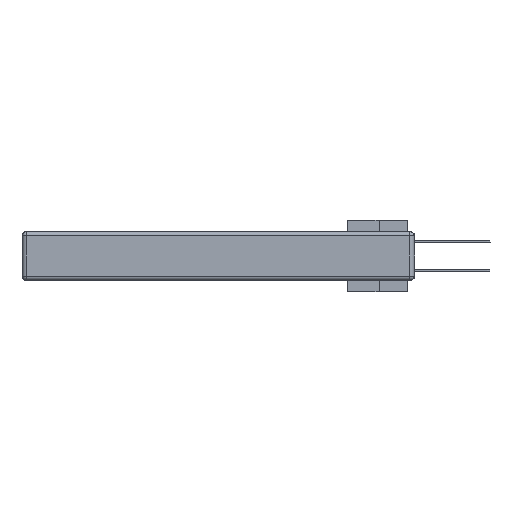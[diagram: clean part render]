
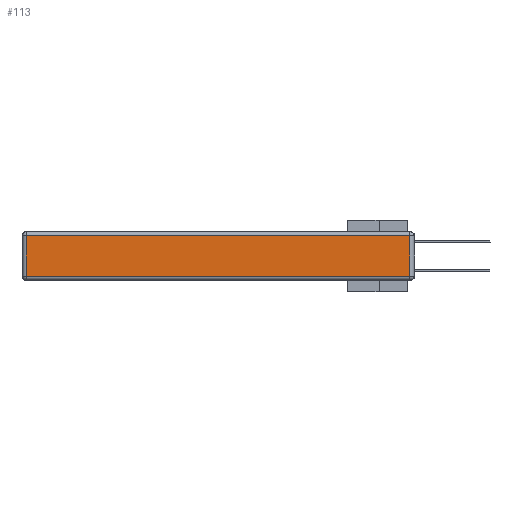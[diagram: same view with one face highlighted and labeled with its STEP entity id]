
A CAD part, left-side view. The second image highlights one B-rep face of the part: STEP entity #113.
In plain terms, the highlighted planar face has unit normal (-1, 0, 0).
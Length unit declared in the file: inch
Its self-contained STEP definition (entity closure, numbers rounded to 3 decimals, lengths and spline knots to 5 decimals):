
#113 = ADVANCED_FACE ( 'NONE', ( #27626 ), #10174, .T. ) ;
#1454 = VERTEX_POINT ( 'NONE', #16090 ) ;
#2201 = AXIS2_PLACEMENT_3D ( 'NONE', #15465, #24579, #2639 ) ;
#2639 = DIRECTION ( 'NONE',  ( 0., 0., 1. ) ) ;
#3125 = DIRECTION ( 'NONE',  ( 0., 0., -1. ) ) ;
#3153 = DIRECTION ( 'NONE',  ( 0., 0., 1. ) ) ;
#3309 = LINE ( 'NONE', #20299, #27949 ) ;
#3883 = CARTESIAN_POINT ( 'NONE',  ( 0., 0.03, -0.03 ) ) ;
#4058 = VERTEX_POINT ( 'NONE', #22180 ) ;
#5304 = ORIENTED_EDGE ( 'NONE', *, *, #15159, .T. ) ;
#5862 = CARTESIAN_POINT ( 'NONE',  ( 0., 2.72, -0.343 ) ) ;
#7704 = CARTESIAN_POINT ( 'NONE',  ( 0., 2.72, -0.313 ) ) ;
#10174 = PLANE ( 'NONE',  #2201 ) ;
#10340 = LINE ( 'NONE', #17716, #16652 ) ;
#10435 = VERTEX_POINT ( 'NONE', #3883 ) ;
#11179 = CARTESIAN_POINT ( 'NONE',  ( 0., 2.75, -0.03 ) ) ;
#12518 = ORIENTED_EDGE ( 'NONE', *, *, #18437, .T. ) ;
#12753 = VECTOR ( 'NONE', #3125, 39.37008 ) ;
#14022 = EDGE_LOOP ( 'NONE', ( #29431, #5304, #17447, #12518 ) ) ;
#14356 = EDGE_CURVE ( 'NONE', #19228, #4058, #10340, .T. ) ;
#15159 = EDGE_CURVE ( 'NONE', #4058, #10435, #3309, .T. ) ;
#15465 = CARTESIAN_POINT ( 'NONE',  ( 0., 0., -0.343 ) ) ;
#16090 = CARTESIAN_POINT ( 'NONE',  ( 0., 2.72, -0.03 ) ) ;
#16652 = VECTOR ( 'NONE', #27465, 39.37008 ) ;
#17447 = ORIENTED_EDGE ( 'NONE', *, *, #31294, .T. ) ;
#17716 = CARTESIAN_POINT ( 'NONE',  ( 0., 0., -0.313 ) ) ;
#18437 = EDGE_CURVE ( 'NONE', #1454, #19228, #22518, .T. ) ;
#19228 = VERTEX_POINT ( 'NONE', #7704 ) ;
#20299 = CARTESIAN_POINT ( 'NONE',  ( 0., 0.03, -0.343 ) ) ;
#22180 = CARTESIAN_POINT ( 'NONE',  ( 0., 0.03, -0.313 ) ) ;
#22518 = LINE ( 'NONE', #5862, #12753 ) ;
#24579 = DIRECTION ( 'NONE',  ( -1., 0., 0. ) ) ;
#27465 = DIRECTION ( 'NONE',  ( 0., -1., 0. ) ) ;
#27626 = FACE_OUTER_BOUND ( 'NONE', #14022, .T. ) ;
#27949 = VECTOR ( 'NONE', #3153, 39.37008 ) ;
#28166 = DIRECTION ( 'NONE',  ( 0., 1., 0. ) ) ;
#28320 = LINE ( 'NONE', #11179, #29915 ) ;
#29431 = ORIENTED_EDGE ( 'NONE', *, *, #14356, .T. ) ;
#29915 = VECTOR ( 'NONE', #28166, 39.37008 ) ;
#31294 = EDGE_CURVE ( 'NONE', #10435, #1454, #28320, .T. ) ;
